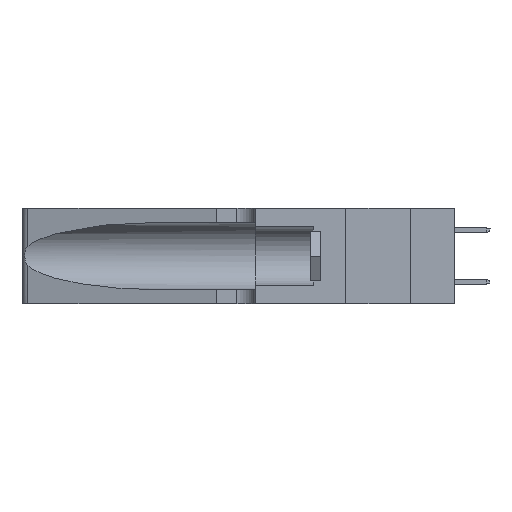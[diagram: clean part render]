
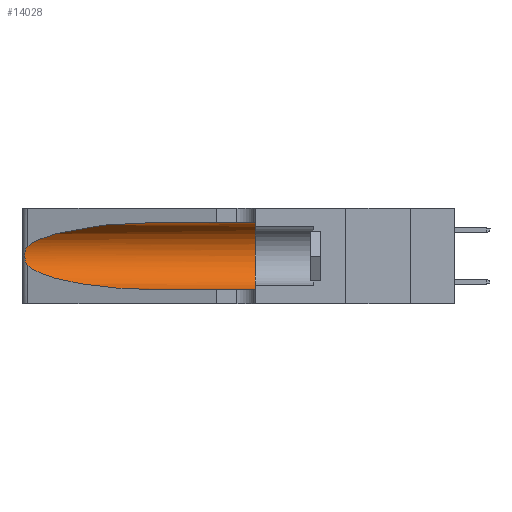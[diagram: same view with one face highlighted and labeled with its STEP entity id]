
A CAD part, left-side view. The second image highlights one B-rep face of the part: STEP entity #14028.
In plain terms, the highlighted cylindrical face has radius 3.308 mm (diameter 6.617 mm), a partial arc.
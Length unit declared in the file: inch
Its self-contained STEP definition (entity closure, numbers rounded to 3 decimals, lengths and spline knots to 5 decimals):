
#233 = EDGE_CURVE ( 'NONE', #16951, #16785, #19630, .T. ) ;
#548 = EDGE_CURVE ( 'NONE', #16785, #3809, #11787, .T. ) ;
#751 = CARTESIAN_POINT ( 'NONE',  ( 0.1305, 0.72297, 0.31525 ) ) ;
#1619 = CARTESIAN_POINT ( 'NONE',  ( 0.1305, 0.35, 0.05475 ) ) ;
#1682 = ORIENTED_EDGE ( 'NONE', *, *, #233, .T. ) ;
#1781 = CARTESIAN_POINT ( 'NONE',  ( 0.25854, 1.2359, 0.20912 ) ) ;
#2200 = ORIENTED_EDGE ( 'NONE', *, *, #6628, .F. ) ;
#2314 = CARTESIAN_POINT ( 'NONE',  ( 0.25555, 1.22993, 0.14849 ) ) ;
#3388 = DIRECTION ( 'NONE',  ( 0., -1., 0. ) ) ;
#3457 =( BOUNDED_CURVE ( )  B_SPLINE_CURVE ( 3, ( #751, #19900, #9521, #17368 ),
 .UNSPECIFIED., .F., .T. ) 
 B_SPLINE_CURVE_WITH_KNOTS ( ( 4, 4 ),
 ( 1.5708, 2.84003 ),
 .UNSPECIFIED. ) 
 CURVE ( )  GEOMETRIC_REPRESENTATION_ITEM ( )  RATIONAL_B_SPLINE_CURVE ( ( 1., 0.87, 0.87, 1. ) ) 
 REPRESENTATION_ITEM ( '' )  );
#3809 = VERTEX_POINT ( 'NONE', #1619 ) ;
#3816 = VECTOR ( 'NONE', #3388, 39.37008 ) ;
#4098 = CARTESIAN_POINT ( 'NONE',  ( 0.1305, 0.72297, 0.31525 ) ) ;
#4255 = ORIENTED_EDGE ( 'NONE', *, *, #26439, .T. ) ;
#4807 = DIRECTION ( 'NONE',  ( 0., -1., 0. ) ) ;
#5649 = CARTESIAN_POINT ( 'NONE',  ( 0.1305, 0.72297, 0.05475 ) ) ;
#6628 = EDGE_CURVE ( 'NONE', #9319, #3809, #26450, .T. ) ;
#7625 = CARTESIAN_POINT ( 'NONE',  ( 0.1305, 1.61858, 0.185 ) ) ;
#7695 = CARTESIAN_POINT ( 'NONE',  ( 0.26075, 1.23896, 0.19203 ) ) ;
#8929 = CARTESIAN_POINT ( 'NONE',  ( 0.1305, 1.61858, 0.05475 ) ) ;
#9319 = VERTEX_POINT ( 'NONE', #11874 ) ;
#9521 = CARTESIAN_POINT ( 'NONE',  ( 0.2373, 1.15595, 0.28018 ) ) ;
#9676 = CARTESIAN_POINT ( 'NONE',  ( 0.26075, 1.23896, 0.178 ) ) ;
#10024 = CARTESIAN_POINT ( 'NONE',  ( 0.25487, 1.22718, 0.14631 ) ) ;
#10033 = CARTESIAN_POINT ( 'NONE',  ( 0.25487, 1.22718, 0.14631 ) ) ;
#11326 = VECTOR ( 'NONE', #4807, 39.37008 ) ;
#11787 = LINE ( 'NONE', #8929, #3816 ) ;
#11874 = CARTESIAN_POINT ( 'NONE',  ( 0.1305, 0.35, 0.31525 ) ) ;
#11898 = EDGE_CURVE ( 'NONE', #29290, #9319, #18378, .T. ) ;
#12666 = ORIENTED_EDGE ( 'NONE', *, *, #31944, .T. ) ;
#12879 = CARTESIAN_POINT ( 'NONE',  ( 0.25787, 1.23484, 0.2124 ) ) ;
#12887 = CARTESIAN_POINT ( 'NONE',  ( 0.2373, 1.15595, 0.08982 ) ) ;
#13239 = CARTESIAN_POINT ( 'NONE',  ( 0.25639, 1.23184, 0.21858 ) ) ;
#13313 = DIRECTION ( 'NONE',  ( 0., 0., 1. ) ) ;
#14028 = ADVANCED_FACE ( 'NONE', ( #29264 ), #34821, .F. ) ;
#14149 = B_SPLINE_CURVE_WITH_KNOTS ( 'NONE', 3,
 ( #32012, #34530, #13239, #12879, #1781, #15366, #7695, #9676, #20561, #15716, #23597, #15541, #2314, #10024 ),
 .UNSPECIFIED., .F., .F.,
 ( 4, 2, 2, 2, 2, 2, 4 ),
 ( 0., 0.00027, 0.00053, 0.00107, 0.0016, 0.00187, 0.00214 ),
 .UNSPECIFIED. ) ;
#15366 = CARTESIAN_POINT ( 'NONE',  ( 0.26018, 1.23835, 0.19895 ) ) ;
#15541 = CARTESIAN_POINT ( 'NONE',  ( 0.25639, 1.23186, 0.15144 ) ) ;
#15716 = CARTESIAN_POINT ( 'NONE',  ( 0.25856, 1.23593, 0.16098 ) ) ;
#16785 = VERTEX_POINT ( 'NONE', #5649 ) ;
#16951 = VERTEX_POINT ( 'NONE', #27972 ) ;
#17368 = CARTESIAN_POINT ( 'NONE',  ( 0.25487, 1.22718, 0.22369 ) ) ;
#17866 = CARTESIAN_POINT ( 'NONE',  ( 0.1305, 0.72297, 0.05475 ) ) ;
#18378 = LINE ( 'NONE', #29308, #11326 ) ;
#18506 = DIRECTION ( 'NONE',  ( 0., -1., 0. ) ) ;
#19630 =( BOUNDED_CURVE ( )  B_SPLINE_CURVE ( 3, ( #10033, #12887, #25934, #17866 ),
 .UNSPECIFIED., .F., .T. ) 
 B_SPLINE_CURVE_WITH_KNOTS ( ( 4, 4 ),
 ( 3.44316, 4.71239 ),
 .UNSPECIFIED. ) 
 CURVE ( )  GEOMETRIC_REPRESENTATION_ITEM ( )  RATIONAL_B_SPLINE_CURVE ( ( 1., 0.87, 0.87, 1. ) ) 
 REPRESENTATION_ITEM ( '' )  );
#19900 = CARTESIAN_POINT ( 'NONE',  ( 0.18966, 0.96281, 0.31525 ) ) ;
#20543 = EDGE_LOOP ( 'NONE', ( #12666, #4255, #1682, #34604, #2200, #30115 ) ) ;
#20561 = CARTESIAN_POINT ( 'NONE',  ( 0.26017, 1.23833, 0.17102 ) ) ;
#22741 = AXIS2_PLACEMENT_3D ( 'NONE', #7625, #18506, #29437 ) ;
#23597 = CARTESIAN_POINT ( 'NONE',  ( 0.25789, 1.23486, 0.15765 ) ) ;
#23958 = VERTEX_POINT ( 'NONE', #34669 ) ;
#25934 = CARTESIAN_POINT ( 'NONE',  ( 0.18966, 0.96281, 0.05475 ) ) ;
#26439 = EDGE_CURVE ( 'NONE', #23958, #16951, #14149, .T. ) ;
#26450 = CIRCLE ( 'NONE', #34458, 0.13025 ) ;
#26709 = DIRECTION ( 'NONE',  ( 0., 1., 0. ) ) ;
#27972 = CARTESIAN_POINT ( 'NONE',  ( 0.25487, 1.22718, 0.14631 ) ) ;
#29264 = FACE_OUTER_BOUND ( 'NONE', #20543, .T. ) ;
#29290 = VERTEX_POINT ( 'NONE', #4098 ) ;
#29308 = CARTESIAN_POINT ( 'NONE',  ( 0.1305, 1.61858, 0.31525 ) ) ;
#29437 = DIRECTION ( 'NONE',  ( 0., 0., -1. ) ) ;
#30115 = ORIENTED_EDGE ( 'NONE', *, *, #11898, .F. ) ;
#31944 = EDGE_CURVE ( 'NONE', #29290, #23958, #3457, .T. ) ;
#32012 = CARTESIAN_POINT ( 'NONE',  ( 0.25487, 1.22718, 0.22369 ) ) ;
#34458 = AXIS2_PLACEMENT_3D ( 'NONE', #34790, #26709, #13313 ) ;
#34530 = CARTESIAN_POINT ( 'NONE',  ( 0.25555, 1.22994, 0.2215 ) ) ;
#34604 = ORIENTED_EDGE ( 'NONE', *, *, #548, .T. ) ;
#34669 = CARTESIAN_POINT ( 'NONE',  ( 0.25487, 1.22718, 0.22369 ) ) ;
#34790 = CARTESIAN_POINT ( 'NONE',  ( 0.1305, 0.35, 0.185 ) ) ;
#34821 = CYLINDRICAL_SURFACE ( 'NONE', #22741, 0.13025 ) ;
